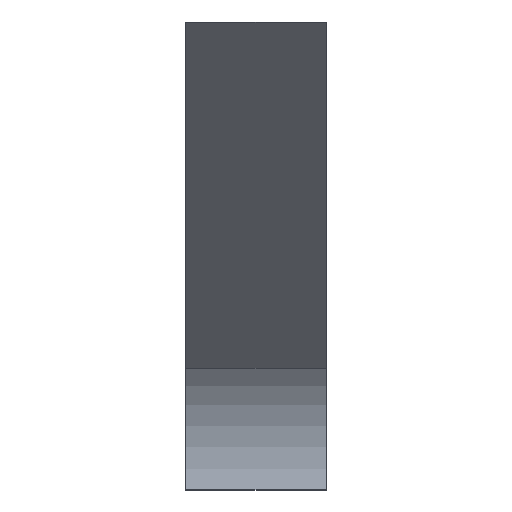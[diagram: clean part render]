
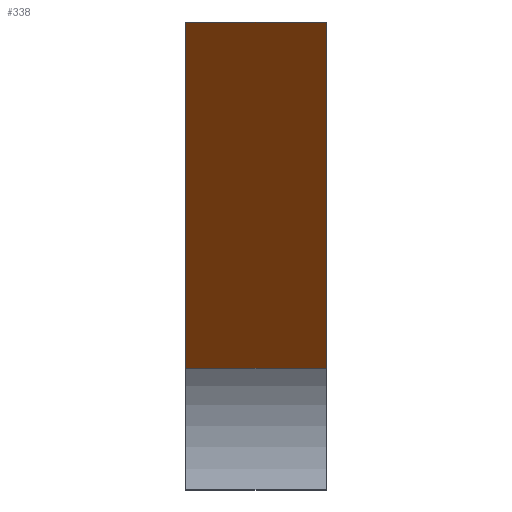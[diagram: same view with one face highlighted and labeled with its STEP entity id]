
A CAD part, top view. The second image highlights one B-rep face of the part: STEP entity #338.
In plain terms, the highlighted planar face has unit normal (0, -0.707, 0.707).
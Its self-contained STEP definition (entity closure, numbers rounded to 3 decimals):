
#16 = CARTESIAN_POINT ( 'NONE',  ( 3.001, -0.732, 0.732 ) ) ;
#17 = LINE ( 'NONE', #283, #387 ) ;
#19 = ORIENTED_EDGE ( 'NONE', *, *, #290, .T. ) ;
#29 = CARTESIAN_POINT ( 'NONE',  ( 3., -0.732, 0.732 ) ) ;
#41 = VERTEX_POINT ( 'NONE', #314 ) ;
#54 = DIRECTION ( 'NONE',  ( 0., 0.707, 0.707 ) ) ;
#76 = DIRECTION ( 'NONE',  ( -1., 0., 0. ) ) ;
#88 = VECTOR ( 'NONE', #418, 1000. ) ;
#89 = CARTESIAN_POINT ( 'NONE',  ( 0., -0.732, 0.732 ) ) ;
#107 = CARTESIAN_POINT ( 'NONE',  ( 0., 0.097, 1.561 ) ) ;
#109 = EDGE_LOOP ( 'NONE', ( #19, #410, #353, #119 ) ) ;
#119 = ORIENTED_EDGE ( 'NONE', *, *, #354, .F. ) ;
#149 = AXIS2_PLACEMENT_3D ( 'NONE', #16, #261, #54 ) ;
#170 = EDGE_CURVE ( 'NONE', #369, #246, #435, .T. ) ;
#183 = LINE ( 'NONE', #324, #88 ) ;
#192 = FACE_OUTER_BOUND ( 'NONE', #109, .T. ) ;
#222 = PLANE ( 'NONE',  #149 ) ;
#231 = DIRECTION ( 'NONE',  ( 0., 0.707, 0.707 ) ) ;
#246 = VERTEX_POINT ( 'NONE', #107 ) ;
#261 = DIRECTION ( 'NONE',  ( 0., 0.707, -0.707 ) ) ;
#268 = CARTESIAN_POINT ( 'NONE',  ( 0., 7.5, 8.964 ) ) ;
#272 = VECTOR ( 'NONE', #334, 1000. ) ;
#283 = CARTESIAN_POINT ( 'NONE',  ( 12.142, 7.5, 8.964 ) ) ;
#290 = EDGE_CURVE ( 'NONE', #340, #41, #309, .T. ) ;
#295 = VECTOR ( 'NONE', #231, 1000. ) ;
#308 = EDGE_CURVE ( 'NONE', #41, #369, #17, .T. ) ;
#309 = LINE ( 'NONE', #29, #295 ) ;
#314 = CARTESIAN_POINT ( 'NONE',  ( 3., 7.5, 8.964 ) ) ;
#324 = CARTESIAN_POINT ( 'NONE',  ( 3.001, 0.097, 1.561 ) ) ;
#334 = DIRECTION ( 'NONE',  ( 0., -0.707, -0.707 ) ) ;
#338 = ADVANCED_FACE ( 'NONE', ( #192 ), #222, .F. ) ;
#340 = VERTEX_POINT ( 'NONE', #427 ) ;
#353 = ORIENTED_EDGE ( 'NONE', *, *, #170, .T. ) ;
#354 = EDGE_CURVE ( 'NONE', #340, #246, #183, .T. ) ;
#369 = VERTEX_POINT ( 'NONE', #268 ) ;
#387 = VECTOR ( 'NONE', #76, 1000. ) ;
#410 = ORIENTED_EDGE ( 'NONE', *, *, #308, .T. ) ;
#418 = DIRECTION ( 'NONE',  ( -1., 0., 0. ) ) ;
#427 = CARTESIAN_POINT ( 'NONE',  ( 3., 0.097, 1.561 ) ) ;
#435 = LINE ( 'NONE', #89, #272 ) ;
